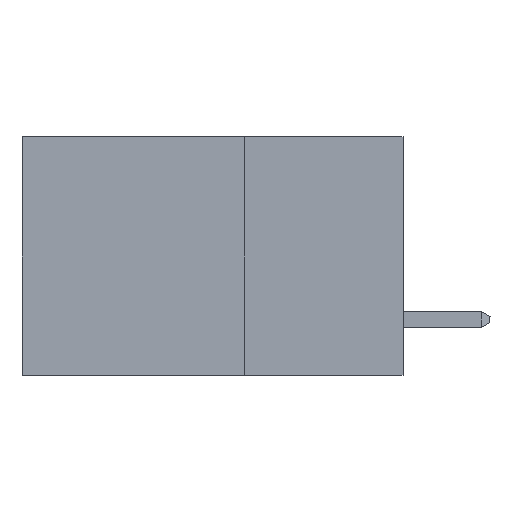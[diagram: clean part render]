
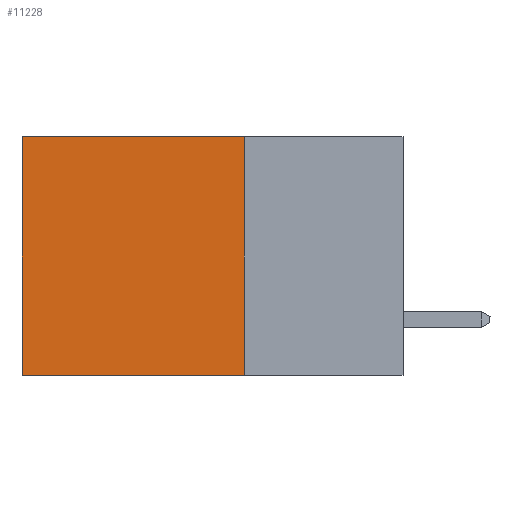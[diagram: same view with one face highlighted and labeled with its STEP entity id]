
A CAD part, left-side view. The second image highlights one B-rep face of the part: STEP entity #11228.
In plain terms, the highlighted planar face has unit normal (-1, 0, 0).
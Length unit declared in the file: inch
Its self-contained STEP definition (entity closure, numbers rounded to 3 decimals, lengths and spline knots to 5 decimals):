
#27 = VERTEX_POINT ( 'NONE', #9972 ) ;
#179 = EDGE_CURVE ( 'NONE', #1632, #4250, #2637, .T. ) ;
#268 = LINE ( 'NONE', #10135, #6262 ) ;
#284 = ORIENTED_EDGE ( 'NONE', *, *, #11515, .F. ) ;
#813 = CARTESIAN_POINT ( 'NONE',  ( 0.2875, 0.6, -0.375 ) ) ;
#826 = VERTEX_POINT ( 'NONE', #6814 ) ;
#886 = VECTOR ( 'NONE', #3704, 39.37008 ) ;
#1419 = CARTESIAN_POINT ( 'NONE',  ( 0.2875, 0.25, -0.375 ) ) ;
#1632 = VERTEX_POINT ( 'NONE', #1834 ) ;
#1719 = VECTOR ( 'NONE', #6217, 39.37008 ) ;
#1834 = CARTESIAN_POINT ( 'NONE',  ( 0.2875, 0.6, 0. ) ) ;
#2150 = CARTESIAN_POINT ( 'NONE',  ( 0.2875, 0.25, 0. ) ) ;
#2637 = LINE ( 'NONE', #5506, #886 ) ;
#2762 = DIRECTION ( 'NONE',  ( 0., 0., -1. ) ) ;
#3160 = EDGE_CURVE ( 'NONE', #27, #4250, #268, .T. ) ;
#3247 = AXIS2_PLACEMENT_3D ( 'NONE', #6953, #12141, #2762 ) ;
#3704 = DIRECTION ( 'NONE',  ( 0., 0., -1. ) ) ;
#4250 = VERTEX_POINT ( 'NONE', #813 ) ;
#4420 = LINE ( 'NONE', #1419, #11751 ) ;
#5120 = ORIENTED_EDGE ( 'NONE', *, *, #9883, .T. ) ;
#5506 = CARTESIAN_POINT ( 'NONE',  ( 0.2875, 0.6, -0.375 ) ) ;
#6217 = DIRECTION ( 'NONE',  ( 0., 1., 0. ) ) ;
#6262 = VECTOR ( 'NONE', #12127, 39.37008 ) ;
#6616 = DIRECTION ( 'NONE',  ( 0., 0., -1. ) ) ;
#6814 = CARTESIAN_POINT ( 'NONE',  ( 0.2875, 0.25, 0. ) ) ;
#6953 = CARTESIAN_POINT ( 'NONE',  ( 0.2875, 0.25, -0.375 ) ) ;
#7211 = LINE ( 'NONE', #2150, #1719 ) ;
#8886 = PLANE ( 'NONE',  #3247 ) ;
#9883 = EDGE_CURVE ( 'NONE', #826, #1632, #7211, .T. ) ;
#9884 = FACE_OUTER_BOUND ( 'NONE', #11918, .T. ) ;
#9972 = CARTESIAN_POINT ( 'NONE',  ( 0.2875, 0.25, -0.375 ) ) ;
#10135 = CARTESIAN_POINT ( 'NONE',  ( 0.2875, 0.25, -0.375 ) ) ;
#10183 = ORIENTED_EDGE ( 'NONE', *, *, #179, .T. ) ;
#11228 = ADVANCED_FACE ( 'NONE', ( #9884 ), #8886, .F. ) ;
#11515 = EDGE_CURVE ( 'NONE', #826, #27, #4420, .T. ) ;
#11751 = VECTOR ( 'NONE', #6616, 39.37008 ) ;
#11918 = EDGE_LOOP ( 'NONE', ( #10183, #11983, #284, #5120 ) ) ;
#11983 = ORIENTED_EDGE ( 'NONE', *, *, #3160, .F. ) ;
#12127 = DIRECTION ( 'NONE',  ( 0., 1., 0. ) ) ;
#12141 = DIRECTION ( 'NONE',  ( 1., 0., 0. ) ) ;
